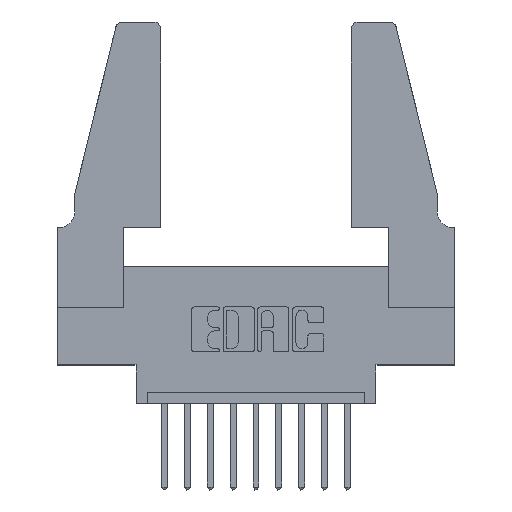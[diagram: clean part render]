
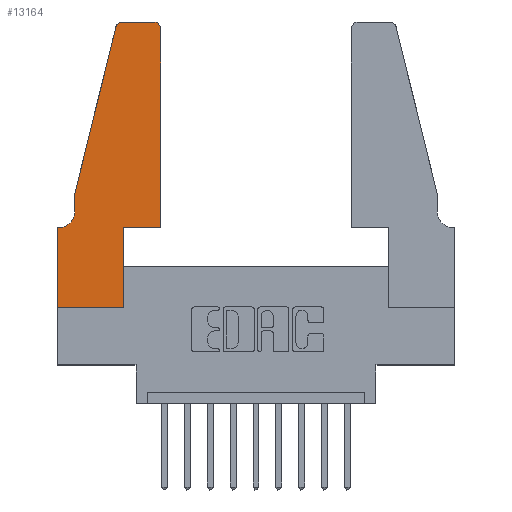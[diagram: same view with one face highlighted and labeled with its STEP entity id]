
A CAD part, top view. The second image highlights one B-rep face of the part: STEP entity #13164.
In plain terms, the highlighted planar face has unit normal (0, 0, 1).
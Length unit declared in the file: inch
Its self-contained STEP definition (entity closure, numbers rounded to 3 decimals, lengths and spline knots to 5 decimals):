
#22 = CARTESIAN_POINT ( 'NONE',  ( 0.4505, 0.35, 0.37 ) ) ;
#40 = VERTEX_POINT ( 'NONE', #12701 ) ;
#147 = DIRECTION ( 'NONE',  ( 1., 0., 0. ) ) ;
#281 = CARTESIAN_POINT ( 'NONE',  ( 0.0055, 0.35, 0.37 ) ) ;
#351 = VERTEX_POINT ( 'NONE', #12485 ) ;
#610 = CIRCLE ( 'NONE', #2676, 0.03 ) ;
#666 = ORIENTED_EDGE ( 'NONE', *, *, #9109, .T. ) ;
#798 = AXIS2_PLACEMENT_3D ( 'NONE', #4356, #11687, #12730 ) ;
#939 = CARTESIAN_POINT ( 'NONE',  ( 0.0755, 0.5, 0.37 ) ) ;
#1110 = CARTESIAN_POINT ( 'NONE',  ( 0., 0.35, 0.37 ) ) ;
#1153 = VERTEX_POINT ( 'NONE', #1110 ) ;
#1252 = CARTESIAN_POINT ( 'NONE',  ( 0., 0., 0.37 ) ) ;
#1309 = VERTEX_POINT ( 'NONE', #1252 ) ;
#1500 = ORIENTED_EDGE ( 'NONE', *, *, #2419, .T. ) ;
#2327 = VERTEX_POINT ( 'NONE', #7518 ) ;
#2365 = VERTEX_POINT ( 'NONE', #5506 ) ;
#2419 = EDGE_CURVE ( 'NONE', #4628, #3493, #3671, .T. ) ;
#2591 = CARTESIAN_POINT ( 'NONE',  ( 0.2605, 1.25, 0.37 ) ) ;
#2676 = AXIS2_PLACEMENT_3D ( 'NONE', #4889, #12222, #4842 ) ;
#3074 = DIRECTION ( 'NONE',  ( 0., 1., 0. ) ) ;
#3491 = VECTOR ( 'NONE', #8216, 39.37008 ) ;
#3493 = VERTEX_POINT ( 'NONE', #6575 ) ;
#3671 = LINE ( 'NONE', #2591, #8742 ) ;
#3677 = CARTESIAN_POINT ( 'NONE',  ( 0.4205, 1.25, 0.37 ) ) ;
#3802 = EDGE_CURVE ( 'NONE', #2327, #6492, #13120, .T. ) ;
#3962 = LINE ( 'NONE', #4918, #9361 ) ;
#4231 = VERTEX_POINT ( 'NONE', #281 ) ;
#4352 = CARTESIAN_POINT ( 'NONE',  ( 0.0755, 0.5, 0.37 ) ) ;
#4356 = CARTESIAN_POINT ( 'NONE',  ( 0.0055, 0.42, 0.37 ) ) ;
#4580 = VERTEX_POINT ( 'NONE', #11664 ) ;
#4628 = VERTEX_POINT ( 'NONE', #3677 ) ;
#4650 = EDGE_CURVE ( 'NONE', #351, #6652, #12627, .T. ) ;
#4675 = AXIS2_PLACEMENT_3D ( 'NONE', #10685, #10732, #147 ) ;
#4712 = EDGE_CURVE ( 'NONE', #6652, #2365, #3962, .T. ) ;
#4842 = DIRECTION ( 'NONE',  ( 1., 0., 0. ) ) ;
#4889 = CARTESIAN_POINT ( 'NONE',  ( 0.4205, 1.22, 0.37 ) ) ;
#4918 = CARTESIAN_POINT ( 'NONE',  ( 0.0755, 0.5, 0.37 ) ) ;
#5275 = DIRECTION ( 'NONE',  ( 1., 0., 0. ) ) ;
#5310 = EDGE_CURVE ( 'NONE', #40, #4580, #11174, .T. ) ;
#5389 = EDGE_CURVE ( 'NONE', #4580, #2327, #5587, .T. ) ;
#5399 = LINE ( 'NONE', #5985, #9669 ) ;
#5506 = CARTESIAN_POINT ( 'NONE',  ( 0.0755, 0.42, 0.37 ) ) ;
#5587 = LINE ( 'NONE', #8380, #8031 ) ;
#5594 = EDGE_LOOP ( 'NONE', ( #1500, #13273, #5789, #8604, #10939, #9313, #9323, #11866, #12172, #12324, #10909, #666 ) ) ;
#5789 = ORIENTED_EDGE ( 'NONE', *, *, #4650, .T. ) ;
#5985 = CARTESIAN_POINT ( 'NONE',  ( 0.0755, 0.35, 0.37 ) ) ;
#6251 = EDGE_CURVE ( 'NONE', #4231, #1153, #5399, .T. ) ;
#6420 = DIRECTION ( 'NONE',  ( 0., 1., 0. ) ) ;
#6492 = VERTEX_POINT ( 'NONE', #7860 ) ;
#6575 = CARTESIAN_POINT ( 'NONE',  ( 0.284, 1.25, 0.37 ) ) ;
#6652 = VERTEX_POINT ( 'NONE', #4352 ) ;
#6817 = VECTOR ( 'NONE', #7323, 39.37008 ) ;
#7041 = DIRECTION ( 'NONE',  ( -1., 0., 0. ) ) ;
#7206 = EDGE_CURVE ( 'NONE', #1153, #1309, #8802, .T. ) ;
#7323 = DIRECTION ( 'NONE',  ( 0., -1., 0. ) ) ;
#7502 = DIRECTION ( 'NONE',  ( 1., 0., 0. ) ) ;
#7518 = CARTESIAN_POINT ( 'NONE',  ( 0.4505, 0.35, 0.37 ) ) ;
#7549 = CARTESIAN_POINT ( 'NONE',  ( 0., 0., 0.37 ) ) ;
#7575 = EDGE_CURVE ( 'NONE', #3493, #351, #8131, .T. ) ;
#7860 = CARTESIAN_POINT ( 'NONE',  ( 0.4505, 1.22, 0.37 ) ) ;
#8031 = VECTOR ( 'NONE', #5275, 39.37008 ) ;
#8116 = DIRECTION ( 'NONE',  ( 0., -1., 0. ) ) ;
#8131 = CIRCLE ( 'NONE', #8866, 0.03 ) ;
#8201 = VECTOR ( 'NONE', #3074, 39.37008 ) ;
#8216 = DIRECTION ( 'NONE',  ( -0.239, -0.971, 0. ) ) ;
#8324 = FACE_OUTER_BOUND ( 'NONE', #5594, .T. ) ;
#8380 = CARTESIAN_POINT ( 'NONE',  ( 0.4505, 0.35, 0.37 ) ) ;
#8604 = ORIENTED_EDGE ( 'NONE', *, *, #4712, .T. ) ;
#8742 = VECTOR ( 'NONE', #12890, 39.37008 ) ;
#8802 = LINE ( 'NONE', #12461, #6817 ) ;
#8866 = AXIS2_PLACEMENT_3D ( 'NONE', #11725, #10842, #12771 ) ;
#8916 = EDGE_CURVE ( 'NONE', #1309, #40, #12058, .T. ) ;
#8926 = VECTOR ( 'NONE', #7502, 39.37008 ) ;
#9109 = EDGE_CURVE ( 'NONE', #6492, #4628, #610, .T. ) ;
#9313 = ORIENTED_EDGE ( 'NONE', *, *, #6251, .T. ) ;
#9323 = ORIENTED_EDGE ( 'NONE', *, *, #7206, .T. ) ;
#9361 = VECTOR ( 'NONE', #8116, 39.37008 ) ;
#9669 = VECTOR ( 'NONE', #7041, 39.37008 ) ;
#10253 = CARTESIAN_POINT ( 'NONE',  ( 0.2865, 0.35, 0.37 ) ) ;
#10685 = CARTESIAN_POINT ( 'NONE',  ( 0., 0.35, 0.37 ) ) ;
#10732 = DIRECTION ( 'NONE',  ( 0., 0., 1. ) ) ;
#10842 = DIRECTION ( 'NONE',  ( 0., 0., 1. ) ) ;
#10909 = ORIENTED_EDGE ( 'NONE', *, *, #3802, .T. ) ;
#10939 = ORIENTED_EDGE ( 'NONE', *, *, #12034, .T. ) ;
#11174 = LINE ( 'NONE', #10253, #8201 ) ;
#11366 = VECTOR ( 'NONE', #6420, 39.37008 ) ;
#11664 = CARTESIAN_POINT ( 'NONE',  ( 0.2865, 0.35, 0.37 ) ) ;
#11687 = DIRECTION ( 'NONE',  ( 0., 0., -1. ) ) ;
#11725 = CARTESIAN_POINT ( 'NONE',  ( 0.284, 1.22, 0.37 ) ) ;
#11866 = ORIENTED_EDGE ( 'NONE', *, *, #8916, .T. ) ;
#12034 = EDGE_CURVE ( 'NONE', #2365, #4231, #12450, .T. ) ;
#12058 = LINE ( 'NONE', #7549, #8926 ) ;
#12172 = ORIENTED_EDGE ( 'NONE', *, *, #5310, .T. ) ;
#12222 = DIRECTION ( 'NONE',  ( 0., 0., 1. ) ) ;
#12324 = ORIENTED_EDGE ( 'NONE', *, *, #5389, .T. ) ;
#12450 = CIRCLE ( 'NONE', #798, 0.07 ) ;
#12461 = CARTESIAN_POINT ( 'NONE',  ( 0., 0., 0.37 ) ) ;
#12485 = CARTESIAN_POINT ( 'NONE',  ( 0.25487, 1.22718, 0.37 ) ) ;
#12627 = LINE ( 'NONE', #939, #3491 ) ;
#12701 = CARTESIAN_POINT ( 'NONE',  ( 0.2865, 0., 0.37 ) ) ;
#12730 = DIRECTION ( 'NONE',  ( -1., 0., 0. ) ) ;
#12771 = DIRECTION ( 'NONE',  ( 1., 0., 0. ) ) ;
#12889 = PLANE ( 'NONE',  #4675 ) ;
#12890 = DIRECTION ( 'NONE',  ( -1., 0., 0. ) ) ;
#13120 = LINE ( 'NONE', #22, #11366 ) ;
#13164 = ADVANCED_FACE ( 'NONE', ( #8324 ), #12889, .T. ) ;
#13273 = ORIENTED_EDGE ( 'NONE', *, *, #7575, .T. ) ;
